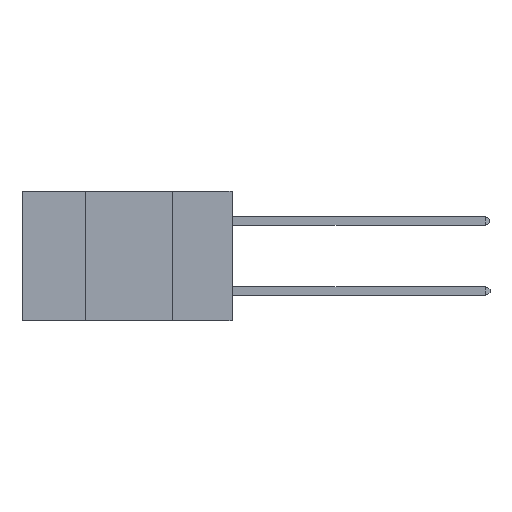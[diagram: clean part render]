
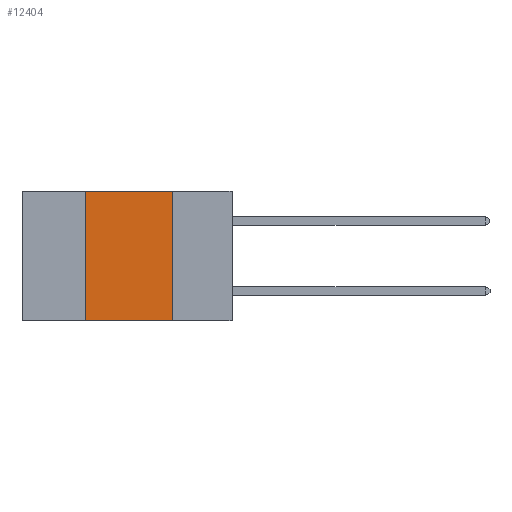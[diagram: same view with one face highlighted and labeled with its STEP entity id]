
A CAD part, left-side view. The second image highlights one B-rep face of the part: STEP entity #12404.
In plain terms, the highlighted planar face has unit normal (-1, 0, 0).
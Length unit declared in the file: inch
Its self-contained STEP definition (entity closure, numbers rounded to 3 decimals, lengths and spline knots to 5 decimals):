
#601 = AXIS2_PLACEMENT_3D ( 'NONE', #7746, #9838, #3283 ) ;
#1724 = CARTESIAN_POINT ( 'NONE',  ( 0., 0.6, 0. ) ) ;
#1811 = ORIENTED_EDGE ( 'NONE', *, *, #9519, .F. ) ;
#1905 = CARTESIAN_POINT ( 'NONE',  ( 0., 0.17, 0. ) ) ;
#2242 = LINE ( 'NONE', #9000, #3815 ) ;
#3094 = CARTESIAN_POINT ( 'NONE',  ( 0., 0.17, 0. ) ) ;
#3281 = LINE ( 'NONE', #1724, #6302 ) ;
#3283 = DIRECTION ( 'NONE',  ( 0., 0., -1. ) ) ;
#3419 = VERTEX_POINT ( 'NONE', #3844 ) ;
#3815 = VECTOR ( 'NONE', #12127, 39.37008 ) ;
#3844 = CARTESIAN_POINT ( 'NONE',  ( 0., 0.42, -0.37 ) ) ;
#3931 = LINE ( 'NONE', #3094, #12795 ) ;
#3986 = DIRECTION ( 'NONE',  ( 0., -1., 0. ) ) ;
#4655 = LINE ( 'NONE', #13256, #10412 ) ;
#5179 = ORIENTED_EDGE ( 'NONE', *, *, #9266, .F. ) ;
#5617 = VERTEX_POINT ( 'NONE', #7807 ) ;
#5719 = EDGE_LOOP ( 'NONE', ( #7455, #1811, #5179, #8122 ) ) ;
#6302 = VECTOR ( 'NONE', #3986, 39.37008 ) ;
#7064 = DIRECTION ( 'NONE',  ( 0., -1., 0. ) ) ;
#7455 = ORIENTED_EDGE ( 'NONE', *, *, #12295, .F. ) ;
#7746 = CARTESIAN_POINT ( 'NONE',  ( 0., 0.6, 0. ) ) ;
#7807 = CARTESIAN_POINT ( 'NONE',  ( 0., 0.17, -0.37 ) ) ;
#8120 = FACE_OUTER_BOUND ( 'NONE', #5719, .T. ) ;
#8122 = ORIENTED_EDGE ( 'NONE', *, *, #11343, .T. ) ;
#8608 = DIRECTION ( 'NONE',  ( 0., 0., -1. ) ) ;
#9000 = CARTESIAN_POINT ( 'NONE',  ( 0., 0.42, 0. ) ) ;
#9266 = EDGE_CURVE ( 'NONE', #3419, #11480, #2242, .T. ) ;
#9420 = CARTESIAN_POINT ( 'NONE',  ( 0., 0.42, 0. ) ) ;
#9519 = EDGE_CURVE ( 'NONE', #11480, #10185, #3281, .T. ) ;
#9838 = DIRECTION ( 'NONE',  ( 1., 0., 0. ) ) ;
#10185 = VERTEX_POINT ( 'NONE', #1905 ) ;
#10412 = VECTOR ( 'NONE', #7064, 39.37008 ) ;
#11343 = EDGE_CURVE ( 'NONE', #3419, #5617, #4655, .T. ) ;
#11480 = VERTEX_POINT ( 'NONE', #9420 ) ;
#11877 = PLANE ( 'NONE',  #601 ) ;
#12127 = DIRECTION ( 'NONE',  ( 0., 0., 1. ) ) ;
#12295 = EDGE_CURVE ( 'NONE', #10185, #5617, #3931, .T. ) ;
#12404 = ADVANCED_FACE ( 'NONE', ( #8120 ), #11877, .F. ) ;
#12795 = VECTOR ( 'NONE', #8608, 39.37008 ) ;
#13256 = CARTESIAN_POINT ( 'NONE',  ( 0., 0.6, -0.37 ) ) ;
